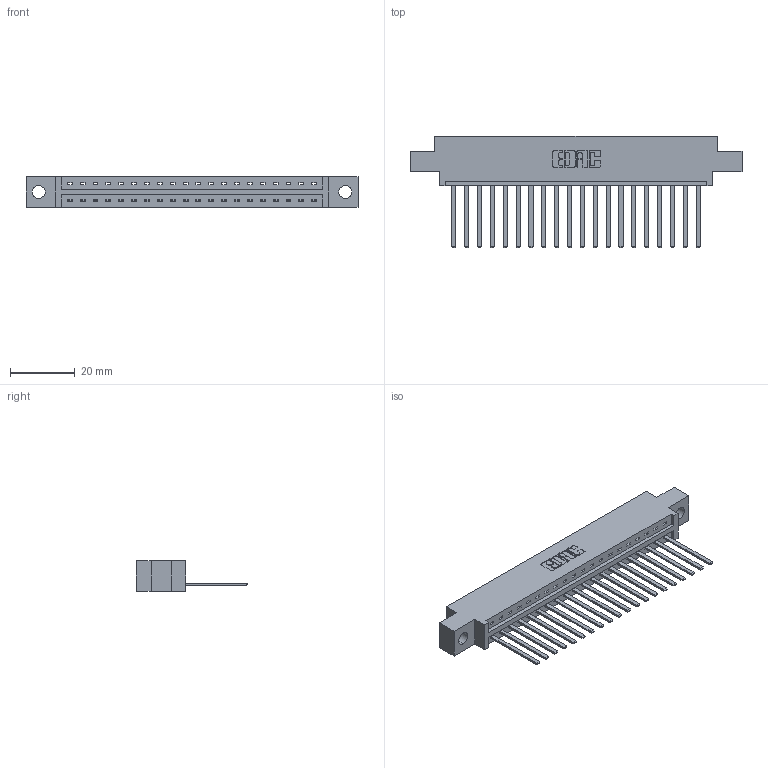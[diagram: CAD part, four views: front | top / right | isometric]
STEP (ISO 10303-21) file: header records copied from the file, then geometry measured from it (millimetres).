
FILE_DESCRIPTION (( 'STEP AP203' ), '1' );
FILE_NAME ('387-020-544-604.STEP', '2019-10-02T23:05:32', ( '' ), ( '' ), 'SwSTEP 2.0', 'SolidWorks 2016', '' );
FILE_SCHEMA (( 'CONFIG_CONTROL_DESIGN' ));
Length unit declared in the file: inch
Products named in the file (3): 387-020-544-604; 345-292-001_345-293-144; 337 Part_0.170 Offset - 0.156 Dia-TH
Assembly tree (21 placements, depth 2):
  387-020-544-604
    337 Part_0.170 Offset - 0.156 Dia-TH
    345-292-001_345-293-144  x20
Bounding box: 102.26 x 34.3 x 9.4 mm (x, y, z)
Volume: 10379.2 mm3; surface area: 11256.9 mm2
Topology: 21 solids, 21 shells, 1238 faces, 3723 edges, 2454 vertices
Faces by surface type: plane 914, cylinder 324
Entity records: 17663 total; most frequent: CARTESIAN_POINT 3082, ORIENTED_EDGE 3038, DIRECTION 2635, EDGE_CURVE 1519, VECTOR 1395, LINE 1395, VERTEX_POINT 1010, AXIS2_PLACEMENT_3D 620
